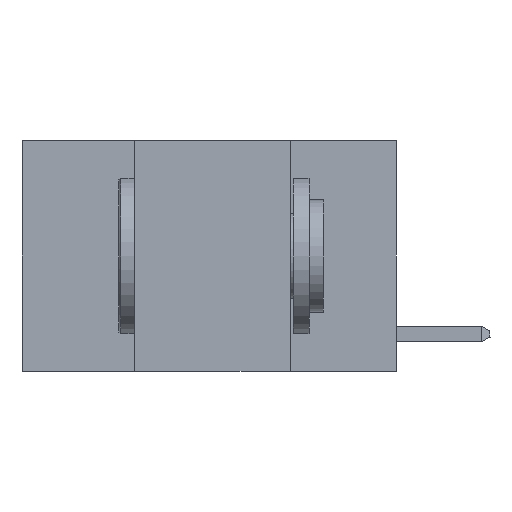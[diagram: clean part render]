
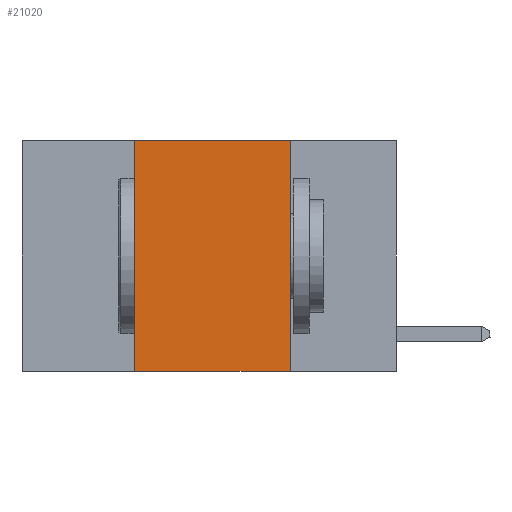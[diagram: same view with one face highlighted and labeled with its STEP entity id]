
A CAD part, left-side view. The second image highlights one B-rep face of the part: STEP entity #21020.
In plain terms, the highlighted planar face has unit normal (-1, 0, 0).
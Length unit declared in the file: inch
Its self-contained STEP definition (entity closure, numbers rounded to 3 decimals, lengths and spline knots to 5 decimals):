
#239 = DIRECTION ( 'NONE',  ( 0., 0., -1. ) ) ;
#933 = CARTESIAN_POINT ( 'NONE',  ( 0., 0.6, 0. ) ) ;
#1029 = LINE ( 'NONE', #933, #6578 ) ;
#1230 = DIRECTION ( 'NONE',  ( 0., 0., -1. ) ) ;
#1969 = CARTESIAN_POINT ( 'NONE',  ( 0., 0.17, 0. ) ) ;
#4398 = EDGE_CURVE ( 'NONE', #16378, #23726, #14183, .T. ) ;
#4938 = LINE ( 'NONE', #24122, #10518 ) ;
#5720 = CARTESIAN_POINT ( 'NONE',  ( 0., 0.17, -0.37 ) ) ;
#6077 = PLANE ( 'NONE',  #9080 ) ;
#6578 = VECTOR ( 'NONE', #15550, 39.37008 ) ;
#6909 = FACE_OUTER_BOUND ( 'NONE', #12012, .T. ) ;
#8536 = CARTESIAN_POINT ( 'NONE',  ( 0., 0.6, -0.37 ) ) ;
#8662 = ORIENTED_EDGE ( 'NONE', *, *, #4398, .T. ) ;
#9080 = AXIS2_PLACEMENT_3D ( 'NONE', #24763, #12396, #239 ) ;
#10406 = DIRECTION ( 'NONE',  ( 0., 0., 1. ) ) ;
#10407 = EDGE_CURVE ( 'NONE', #14814, #22863, #1029, .T. ) ;
#10429 = CARTESIAN_POINT ( 'NONE',  ( 0., 0.42, -0.37 ) ) ;
#10518 = VECTOR ( 'NONE', #1230, 39.37008 ) ;
#11389 = EDGE_CURVE ( 'NONE', #16378, #14814, #25374, .T. ) ;
#12012 = EDGE_LOOP ( 'NONE', ( #22134, #18647, #17495, #8662 ) ) ;
#12396 = DIRECTION ( 'NONE',  ( 1., 0., 0. ) ) ;
#13509 = VECTOR ( 'NONE', #14758, 39.37008 ) ;
#13969 = CARTESIAN_POINT ( 'NONE',  ( 0., 0.42, 0. ) ) ;
#14183 = LINE ( 'NONE', #8536, #13509 ) ;
#14758 = DIRECTION ( 'NONE',  ( 0., -1., 0. ) ) ;
#14814 = VERTEX_POINT ( 'NONE', #13969 ) ;
#15550 = DIRECTION ( 'NONE',  ( 0., -1., 0. ) ) ;
#16378 = VERTEX_POINT ( 'NONE', #10429 ) ;
#17307 = EDGE_CURVE ( 'NONE', #22863, #23726, #4938, .T. ) ;
#17495 = ORIENTED_EDGE ( 'NONE', *, *, #11389, .F. ) ;
#18647 = ORIENTED_EDGE ( 'NONE', *, *, #10407, .F. ) ;
#21020 = ADVANCED_FACE ( 'NONE', ( #6909 ), #6077, .F. ) ;
#21202 = VECTOR ( 'NONE', #10406, 39.37008 ) ;
#22134 = ORIENTED_EDGE ( 'NONE', *, *, #17307, .F. ) ;
#22790 = CARTESIAN_POINT ( 'NONE',  ( 0., 0.42, 0. ) ) ;
#22863 = VERTEX_POINT ( 'NONE', #1969 ) ;
#23726 = VERTEX_POINT ( 'NONE', #5720 ) ;
#24122 = CARTESIAN_POINT ( 'NONE',  ( 0., 0.17, 0. ) ) ;
#24763 = CARTESIAN_POINT ( 'NONE',  ( 0., 0.6, 0. ) ) ;
#25374 = LINE ( 'NONE', #22790, #21202 ) ;
